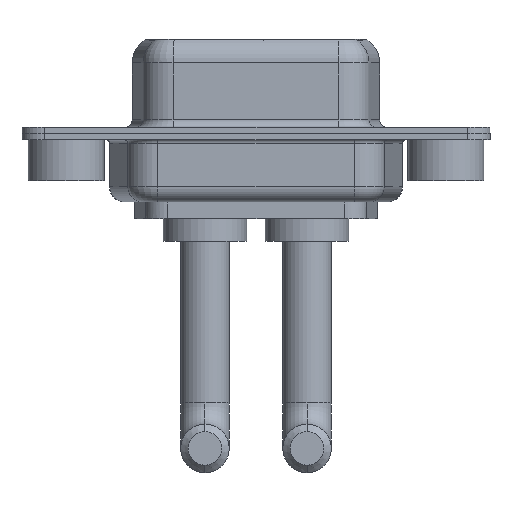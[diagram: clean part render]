
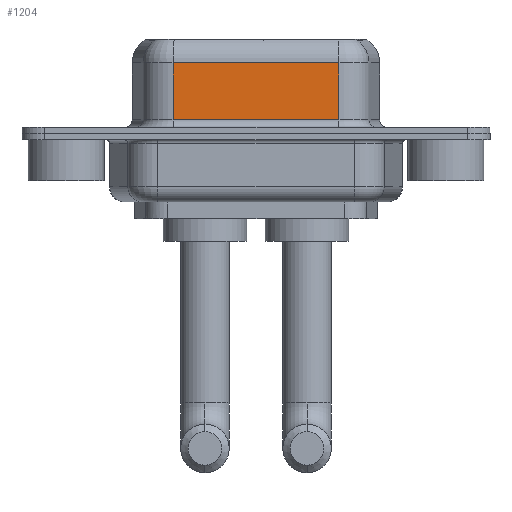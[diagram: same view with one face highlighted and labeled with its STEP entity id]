
A CAD part, front view. The second image highlights one B-rep face of the part: STEP entity #1204.
In plain terms, the highlighted planar face has unit normal (0, -1, 0).
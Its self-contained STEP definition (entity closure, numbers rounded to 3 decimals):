
#84 = DIRECTION ( 'NONE',  ( -1., 0., 0. ) ) ;
#307 = EDGE_CURVE ( 'NONE', #3619, #6004, #4213, .T. ) ;
#413 = CARTESIAN_POINT ( 'NONE',  ( 7.038, -3.95, 6.4 ) ) ;
#429 = DIRECTION ( 'NONE',  ( 0., 1., 0. ) ) ;
#570 = PLANE ( 'NONE',  #8881 ) ;
#1087 = EDGE_CURVE ( 'NONE', #4751, #6004, #3235, .T. ) ;
#1204 = ADVANCED_FACE ( 'NONE', ( #11706 ), #570, .F. ) ;
#1498 = CARTESIAN_POINT ( 'NONE',  ( 17.962, -3.95, 0.9 ) ) ;
#1758 = ORIENTED_EDGE ( 'NONE', *, *, #2238, .T. ) ;
#1865 = EDGE_LOOP ( 'NONE', ( #9884, #13125, #1758, #4333 ) ) ;
#2238 = EDGE_CURVE ( 'NONE', #12091, #3619, #3535, .T. ) ;
#3235 = LINE ( 'NONE', #6181, #11649 ) ;
#3535 = LINE ( 'NONE', #413, #13192 ) ;
#3619 = VERTEX_POINT ( 'NONE', #4301 ) ;
#3718 = CARTESIAN_POINT ( 'NONE',  ( 7.038, -3.95, 4.65 ) ) ;
#3966 = VECTOR ( 'NONE', #4408, 1000. ) ;
#4213 = LINE ( 'NONE', #1498, #3966 ) ;
#4301 = CARTESIAN_POINT ( 'NONE',  ( 7.038, -3.95, 0.9 ) ) ;
#4333 = ORIENTED_EDGE ( 'NONE', *, *, #307, .T. ) ;
#4408 = DIRECTION ( 'NONE',  ( 1., 0., 0. ) ) ;
#4751 = VERTEX_POINT ( 'NONE', #5779 ) ;
#5426 = CARTESIAN_POINT ( 'NONE',  ( 17.962, -3.95, 4.65 ) ) ;
#5602 = EDGE_CURVE ( 'NONE', #4751, #12091, #12445, .T. ) ;
#5779 = CARTESIAN_POINT ( 'NONE',  ( 17.962, -3.95, 4.65 ) ) ;
#6000 = VECTOR ( 'NONE', #84, 1000. ) ;
#6004 = VERTEX_POINT ( 'NONE', #10672 ) ;
#6181 = CARTESIAN_POINT ( 'NONE',  ( 17.962, -3.95, 6.4 ) ) ;
#7422 = DIRECTION ( 'NONE',  ( 0., 0., -1. ) ) ;
#8881 = AXIS2_PLACEMENT_3D ( 'NONE', #12587, #429, #10642 ) ;
#9884 = ORIENTED_EDGE ( 'NONE', *, *, #1087, .F. ) ;
#10642 = DIRECTION ( 'NONE',  ( -1., 0., 0. ) ) ;
#10672 = CARTESIAN_POINT ( 'NONE',  ( 17.962, -3.95, 0.9 ) ) ;
#11517 = DIRECTION ( 'NONE',  ( 0., 0., -1. ) ) ;
#11649 = VECTOR ( 'NONE', #11517, 1000. ) ;
#11706 = FACE_OUTER_BOUND ( 'NONE', #1865, .T. ) ;
#12091 = VERTEX_POINT ( 'NONE', #3718 ) ;
#12445 = LINE ( 'NONE', #5426, #6000 ) ;
#12587 = CARTESIAN_POINT ( 'NONE',  ( 17.962, -3.95, 6.4 ) ) ;
#13125 = ORIENTED_EDGE ( 'NONE', *, *, #5602, .T. ) ;
#13192 = VECTOR ( 'NONE', #7422, 1000. ) ;
